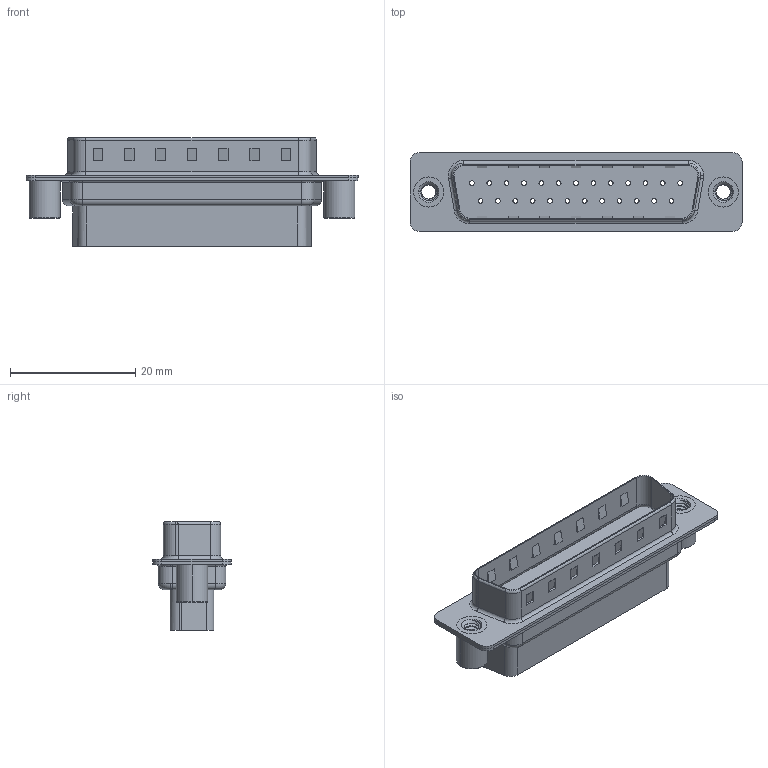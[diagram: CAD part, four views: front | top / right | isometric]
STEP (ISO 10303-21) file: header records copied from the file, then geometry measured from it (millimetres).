
FILE_DESCRIPTION (( 'STEP AP203' ), '1' );
FILE_NAME ('627-025-010-049.STEP', '2020-07-15T20:37:40', ( '' ), ( '' ), 'SwSTEP 2.0', 'SolidWorks 2020', '' );
FILE_SCHEMA (( 'CONFIG_CONTROL_DESIGN' ));
Length unit declared in the file: millimetre
Products named in the file (5): 627 Shell Rear_25 Contacts; 627 Housing_25 HP; 627 Shell Front_25 Contacts; 627-025-010-049; 627 4-40 Threaded Standoff BS
Assembly tree (5 placements, depth 2):
  627-025-010-049
    627 Housing_25 HP
    627 Shell Front_25 Contacts
    627 Shell Rear_25 Contacts
    627 4-40 Threaded Standoff BS  x2
Bounding box: 53 x 12.6 x 17.4 mm (x, y, z)
Volume: 3602.2 mm3; surface area: 6809.1 mm2
Topology: 5 solids, 5 shells, 598 faces, 1471 edges, 944 vertices
Faces by surface type: cylinder 307, plane 221, torus 50, cone 14, bspline 6
Entity records: 18747 total; most frequent: CARTESIAN_POINT 4578, DIRECTION 2999, ORIENTED_EDGE 2716, EDGE_CURVE 1358, AXIS2_PLACEMENT_3D 1149, VERTEX_POINT 871, EDGE_LOOP 705, VECTOR 701
